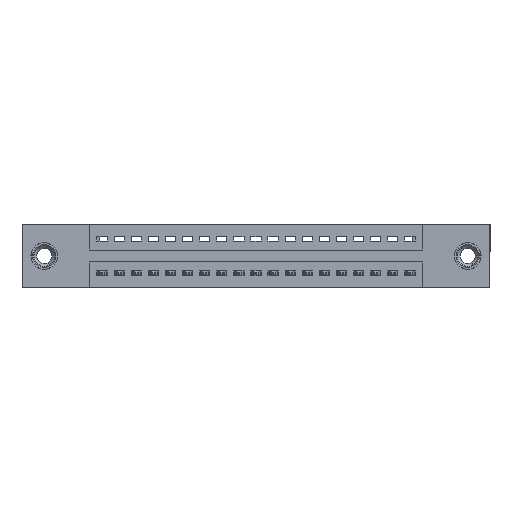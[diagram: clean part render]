
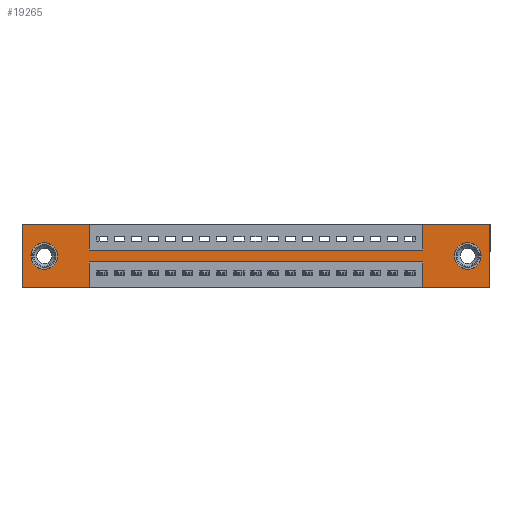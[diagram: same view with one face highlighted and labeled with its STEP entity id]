
A CAD part, front view. The second image highlights one B-rep face of the part: STEP entity #19265.
In plain terms, the highlighted planar face has unit normal (0, -1, 0).
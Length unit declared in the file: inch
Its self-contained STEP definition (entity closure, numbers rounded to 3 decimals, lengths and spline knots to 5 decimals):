
#86 = DIRECTION ( 'NONE',  ( 1., 0., 0. ) ) ;
#312 = VERTEX_POINT ( 'NONE', #5133 ) ;
#320 = CARTESIAN_POINT ( 'NONE',  ( 0., 0., 0. ) ) ;
#334 = DIRECTION ( 'NONE',  ( 0., 0., -1. ) ) ;
#441 = DIRECTION ( 'NONE',  ( 0., 0., -1. ) ) ;
#544 = AXIS2_PLACEMENT_3D ( 'NONE', #1168, #11820, #2863 ) ;
#595 = DIRECTION ( 'NONE',  ( 0., 1., 0. ) ) ;
#657 = CARTESIAN_POINT ( 'NONE',  ( 0.13, 0., -0.185 ) ) ;
#967 = EDGE_CURVE ( 'NONE', #13375, #312, #2102, .T. ) ;
#998 = EDGE_CURVE ( 'NONE', #10227, #14404, #9924, .T. ) ;
#1022 = VECTOR ( 'NONE', #441, 39.37008 ) ;
#1168 = CARTESIAN_POINT ( 'NONE',  ( 2.605, 0., -0.185 ) ) ;
#1196 = LINE ( 'NONE', #3326, #9505 ) ;
#1624 = AXIS2_PLACEMENT_3D ( 'NONE', #10804, #10737, #15391 ) ;
#1871 = VECTOR ( 'NONE', #16895, 39.37008 ) ;
#2102 = LINE ( 'NONE', #7909, #4256 ) ;
#2358 = VERTEX_POINT ( 'NONE', #10020 ) ;
#2504 = VERTEX_POINT ( 'NONE', #15116 ) ;
#2863 = DIRECTION ( 'NONE',  ( 0., 0., -1. ) ) ;
#2984 = CARTESIAN_POINT ( 'NONE',  ( 0., 0., 0. ) ) ;
#3059 = DIRECTION ( 'NONE',  ( 0., 0., -1. ) ) ;
#3318 = ORIENTED_EDGE ( 'NONE', *, *, #3422, .T. ) ;
#3326 = CARTESIAN_POINT ( 'NONE',  ( 2.3425, 0., 0. ) ) ;
#3355 = LINE ( 'NONE', #11943, #17947 ) ;
#3400 = ORIENTED_EDGE ( 'NONE', *, *, #17847, .F. ) ;
#3422 = EDGE_CURVE ( 'NONE', #16237, #4677, #15688, .T. ) ;
#3571 = VERTEX_POINT ( 'NONE', #13221 ) ;
#3620 = CARTESIAN_POINT ( 'NONE',  ( 2.3425, 0., 0. ) ) ;
#3812 = EDGE_CURVE ( 'NONE', #8261, #10227, #11429, .T. ) ;
#4047 = DIRECTION ( 'NONE',  ( -1., 0., 0. ) ) ;
#4256 = VECTOR ( 'NONE', #18480, 39.37008 ) ;
#4677 = VERTEX_POINT ( 'NONE', #12207 ) ;
#4851 = LINE ( 'NONE', #18739, #1022 ) ;
#5133 = CARTESIAN_POINT ( 'NONE',  ( 0.3925, 0., -0.15 ) ) ;
#5177 = DIRECTION ( 'NONE',  ( 1., 0., 0. ) ) ;
#5467 = FACE_BOUND ( 'NONE', #6799, .T. ) ;
#5806 = VECTOR ( 'NONE', #6328, 39.37008 ) ;
#5836 = CARTESIAN_POINT ( 'NONE',  ( 2.605, 0., -0.263 ) ) ;
#5941 = FACE_OUTER_BOUND ( 'NONE', #17268, .T. ) ;
#6328 = DIRECTION ( 'NONE',  ( 1., 0., 0. ) ) ;
#6513 = EDGE_CURVE ( 'NONE', #7461, #15294, #11846, .T. ) ;
#6676 = VECTOR ( 'NONE', #16817, 39.37008 ) ;
#6799 = EDGE_LOOP ( 'NONE', ( #16247, #10869 ) ) ;
#6816 = CARTESIAN_POINT ( 'NONE',  ( 0.3925, 0., -0.22 ) ) ;
#7008 = VECTOR ( 'NONE', #17131, 39.37008 ) ;
#7461 = VERTEX_POINT ( 'NONE', #7712 ) ;
#7576 = FACE_BOUND ( 'NONE', #11920, .T. ) ;
#7712 = CARTESIAN_POINT ( 'NONE',  ( 2.3425, 0., -0.37 ) ) ;
#7909 = CARTESIAN_POINT ( 'NONE',  ( 0.3925, 0., 0. ) ) ;
#8070 = ORIENTED_EDGE ( 'NONE', *, *, #17004, .F. ) ;
#8261 = VERTEX_POINT ( 'NONE', #3620 ) ;
#8644 = ORIENTED_EDGE ( 'NONE', *, *, #3812, .F. ) ;
#8907 = LINE ( 'NONE', #18783, #18068 ) ;
#8968 = VECTOR ( 'NONE', #18726, 39.37008 ) ;
#9017 = EDGE_CURVE ( 'NONE', #312, #13093, #8907, .T. ) ;
#9071 = PLANE ( 'NONE',  #9701 ) ;
#9228 = ORIENTED_EDGE ( 'NONE', *, *, #19479, .F. ) ;
#9254 = DIRECTION ( 'NONE',  ( -1., 0., 0. ) ) ;
#9366 = CARTESIAN_POINT ( 'NONE',  ( 0.3925, 0., 0. ) ) ;
#9426 = LINE ( 'NONE', #2984, #13657 ) ;
#9505 = VECTOR ( 'NONE', #14885, 39.37008 ) ;
#9561 = DIRECTION ( 'NONE',  ( 0., 1., 0. ) ) ;
#9606 = CARTESIAN_POINT ( 'NONE',  ( 2.735, 0., -0.37 ) ) ;
#9651 = CARTESIAN_POINT ( 'NONE',  ( 2.735, 0., 0. ) ) ;
#9701 = AXIS2_PLACEMENT_3D ( 'NONE', #10647, #12015, #3059 ) ;
#9772 = CARTESIAN_POINT ( 'NONE',  ( 0., 0., 0. ) ) ;
#9924 = LINE ( 'NONE', #12208, #1871 ) ;
#9934 = EDGE_CURVE ( 'NONE', #14774, #2358, #4851, .T. ) ;
#10020 = CARTESIAN_POINT ( 'NONE',  ( 0.3925, 0., -0.37 ) ) ;
#10152 = LINE ( 'NONE', #9772, #8968 ) ;
#10227 = VERTEX_POINT ( 'NONE', #9651 ) ;
#10447 = AXIS2_PLACEMENT_3D ( 'NONE', #18712, #595, #334 ) ;
#10563 = CARTESIAN_POINT ( 'NONE',  ( 2.3425, 0., -0.22 ) ) ;
#10647 = CARTESIAN_POINT ( 'NONE',  ( 0., 0., -0.37 ) ) ;
#10703 = ORIENTED_EDGE ( 'NONE', *, *, #15494, .F. ) ;
#10737 = DIRECTION ( 'NONE',  ( 0., 1., 0. ) ) ;
#10804 = CARTESIAN_POINT ( 'NONE',  ( 0.13, 0., -0.185 ) ) ;
#10869 = ORIENTED_EDGE ( 'NONE', *, *, #18036, .T. ) ;
#10992 = LINE ( 'NONE', #6816, #7008 ) ;
#11295 = AXIS2_PLACEMENT_3D ( 'NONE', #657, #9561, #12572 ) ;
#11350 = LINE ( 'NONE', #11613, #12060 ) ;
#11429 = LINE ( 'NONE', #320, #5806 ) ;
#11433 = ORIENTED_EDGE ( 'NONE', *, *, #9934, .F. ) ;
#11613 = CARTESIAN_POINT ( 'NONE',  ( 0., 0., -0.37 ) ) ;
#11820 = DIRECTION ( 'NONE',  ( 0., 1., 0. ) ) ;
#11846 = LINE ( 'NONE', #15361, #6676 ) ;
#11920 = EDGE_LOOP ( 'NONE', ( #3318, #13724 ) ) ;
#11943 = CARTESIAN_POINT ( 'NONE',  ( 0., 0., -0.37 ) ) ;
#12015 = DIRECTION ( 'NONE',  ( 0., -1., 0. ) ) ;
#12060 = VECTOR ( 'NONE', #4047, 39.37008 ) ;
#12108 = CARTESIAN_POINT ( 'NONE',  ( 0.3925, 0., -0.22 ) ) ;
#12207 = CARTESIAN_POINT ( 'NONE',  ( 0.13, 0., -0.263 ) ) ;
#12208 = CARTESIAN_POINT ( 'NONE',  ( 2.735, 0., 0. ) ) ;
#12249 = ORIENTED_EDGE ( 'NONE', *, *, #17379, .F. ) ;
#12515 = CIRCLE ( 'NONE', #10447, 0.078 ) ;
#12572 = DIRECTION ( 'NONE',  ( 0., 0., 1. ) ) ;
#12842 = EDGE_CURVE ( 'NONE', #4677, #16237, #13430, .T. ) ;
#12970 = CIRCLE ( 'NONE', #544, 0.078 ) ;
#13093 = VERTEX_POINT ( 'NONE', #19069 ) ;
#13221 = CARTESIAN_POINT ( 'NONE',  ( 0., 0., -0.37 ) ) ;
#13375 = VERTEX_POINT ( 'NONE', #9366 ) ;
#13430 = CIRCLE ( 'NONE', #1624, 0.078 ) ;
#13657 = VECTOR ( 'NONE', #86, 39.37008 ) ;
#13724 = ORIENTED_EDGE ( 'NONE', *, *, #12842, .T. ) ;
#13758 = EDGE_CURVE ( 'NONE', #2504, #13375, #9426, .T. ) ;
#13924 = ORIENTED_EDGE ( 'NONE', *, *, #998, .F. ) ;
#14262 = VERTEX_POINT ( 'NONE', #15620 ) ;
#14404 = VERTEX_POINT ( 'NONE', #9606 ) ;
#14774 = VERTEX_POINT ( 'NONE', #12108 ) ;
#14885 = DIRECTION ( 'NONE',  ( 0., 0., 1. ) ) ;
#14942 = CARTESIAN_POINT ( 'NONE',  ( 0.13, 0., -0.107 ) ) ;
#15116 = CARTESIAN_POINT ( 'NONE',  ( 0., 0., 0. ) ) ;
#15294 = VERTEX_POINT ( 'NONE', #10563 ) ;
#15361 = CARTESIAN_POINT ( 'NONE',  ( 2.3425, 0., -0.37 ) ) ;
#15391 = DIRECTION ( 'NONE',  ( 0., 0., 1. ) ) ;
#15494 = EDGE_CURVE ( 'NONE', #15294, #14774, #10992, .T. ) ;
#15620 = CARTESIAN_POINT ( 'NONE',  ( 2.605, 0., -0.107 ) ) ;
#15688 = CIRCLE ( 'NONE', #11295, 0.078 ) ;
#16058 = ORIENTED_EDGE ( 'NONE', *, *, #6513, .F. ) ;
#16237 = VERTEX_POINT ( 'NONE', #14942 ) ;
#16247 = ORIENTED_EDGE ( 'NONE', *, *, #19040, .T. ) ;
#16600 = VERTEX_POINT ( 'NONE', #5836 ) ;
#16817 = DIRECTION ( 'NONE',  ( 0., 0., 1. ) ) ;
#16895 = DIRECTION ( 'NONE',  ( 0., 0., -1. ) ) ;
#17004 = EDGE_CURVE ( 'NONE', #13093, #8261, #1196, .T. ) ;
#17131 = DIRECTION ( 'NONE',  ( -1., 0., 0. ) ) ;
#17268 = EDGE_LOOP ( 'NONE', ( #11433, #10703, #16058, #3400, #13924, #8644, #8070, #17837, #18047, #18322, #9228, #12249 ) ) ;
#17379 = EDGE_CURVE ( 'NONE', #2358, #3571, #3355, .T. ) ;
#17837 = ORIENTED_EDGE ( 'NONE', *, *, #9017, .F. ) ;
#17847 = EDGE_CURVE ( 'NONE', #14404, #7461, #11350, .T. ) ;
#17947 = VECTOR ( 'NONE', #9254, 39.37008 ) ;
#18036 = EDGE_CURVE ( 'NONE', #16600, #14262, #12515, .T. ) ;
#18047 = ORIENTED_EDGE ( 'NONE', *, *, #967, .F. ) ;
#18068 = VECTOR ( 'NONE', #5177, 39.37008 ) ;
#18322 = ORIENTED_EDGE ( 'NONE', *, *, #13758, .F. ) ;
#18480 = DIRECTION ( 'NONE',  ( 0., 0., -1. ) ) ;
#18712 = CARTESIAN_POINT ( 'NONE',  ( 2.605, 0., -0.185 ) ) ;
#18726 = DIRECTION ( 'NONE',  ( 0., 0., 1. ) ) ;
#18739 = CARTESIAN_POINT ( 'NONE',  ( 0.3925, 0., -0.37 ) ) ;
#18783 = CARTESIAN_POINT ( 'NONE',  ( 0.3925, 0., -0.15 ) ) ;
#19040 = EDGE_CURVE ( 'NONE', #14262, #16600, #12970, .T. ) ;
#19069 = CARTESIAN_POINT ( 'NONE',  ( 2.3425, 0., -0.15 ) ) ;
#19265 = ADVANCED_FACE ( 'NONE', ( #5467, #7576, #5941 ), #9071, .T. ) ;
#19479 = EDGE_CURVE ( 'NONE', #3571, #2504, #10152, .T. ) ;
